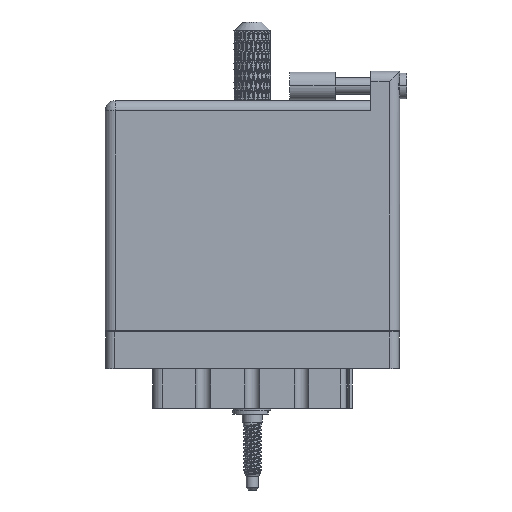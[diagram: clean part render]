
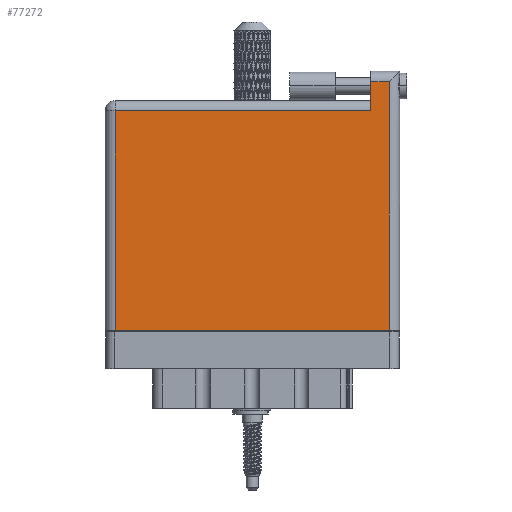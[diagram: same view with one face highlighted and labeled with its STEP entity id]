
A CAD part, front view. The second image highlights one B-rep face of the part: STEP entity #77272.
In plain terms, the highlighted face is planar.
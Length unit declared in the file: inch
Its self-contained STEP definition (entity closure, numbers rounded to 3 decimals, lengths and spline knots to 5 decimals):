
#939 = DIRECTION ( 'NONE',  ( 0., 0., -1. ) ) ;
#3342 = VECTOR ( 'NONE', #53919, 39.37008 ) ;
#4676 = VERTEX_POINT ( 'NONE', #93800 ) ;
#5300 = VERTEX_POINT ( 'NONE', #86890 ) ;
#16044 = ORIENTED_EDGE ( 'NONE', *, *, #45468, .T. ) ;
#17579 = EDGE_CURVE ( 'NONE', #5300, #91844, #90016, .T. ) ;
#21629 = VECTOR ( 'NONE', #67604, 39.37008 ) ;
#21723 = CARTESIAN_POINT ( 'NONE',  ( 1.811, 1.766, 0. ) ) ;
#23541 = VERTEX_POINT ( 'NONE', #57337 ) ;
#26443 = CARTESIAN_POINT ( 'NONE',  ( 0., 1.496, 0. ) ) ;
#26469 = VERTEX_POINT ( 'NONE', #27740 ) ;
#27039 = LINE ( 'NONE', #78316, #68382 ) ;
#27740 = CARTESIAN_POINT ( 'NONE',  ( 0.07, 0., 0. ) ) ;
#29326 = CARTESIAN_POINT ( 'NONE',  ( 0., 1.696, 0. ) ) ;
#29629 = FACE_OUTER_BOUND ( 'NONE', #103637, .T. ) ;
#32016 = ORIENTED_EDGE ( 'NONE', *, *, #65573, .T. ) ;
#35301 = LINE ( 'NONE', #66082, #44280 ) ;
#35376 = ORIENTED_EDGE ( 'NONE', *, *, #35683, .T. ) ;
#35683 = EDGE_CURVE ( 'NONE', #26469, #58102, #27039, .T. ) ;
#37629 = DIRECTION ( 'NONE',  ( -1., 0., 0. ) ) ;
#37657 = CARTESIAN_POINT ( 'NONE',  ( 1.938, 1.766, 0. ) ) ;
#44280 = VECTOR ( 'NONE', #48787, 39.37008 ) ;
#45468 = EDGE_CURVE ( 'NONE', #58102, #23541, #62739, .T. ) ;
#48787 = DIRECTION ( 'NONE',  ( 0., -1., 0. ) ) ;
#49992 = DIRECTION ( 'NONE',  ( -1., 0., 0. ) ) ;
#53919 = DIRECTION ( 'NONE',  ( 0., 1., 0. ) ) ;
#54588 = DIRECTION ( 'NONE',  ( 1., 0., 0. ) ) ;
#56483 = LINE ( 'NONE', #26443, #21629 ) ;
#57337 = CARTESIAN_POINT ( 'NONE',  ( 1.938, 1.696, 0. ) ) ;
#58102 = VERTEX_POINT ( 'NONE', #71157 ) ;
#62739 = LINE ( 'NONE', #37657, #3342 ) ;
#65550 = LINE ( 'NONE', #29326, #77062 ) ;
#65573 = EDGE_CURVE ( 'NONE', #4676, #26469, #35301, .T. ) ;
#66082 = CARTESIAN_POINT ( 'NONE',  ( 0.07, 0., 0. ) ) ;
#66584 = PLANE ( 'NONE',  #104550 ) ;
#67279 = CARTESIAN_POINT ( 'NONE',  ( 0., 1.566, 0. ) ) ;
#67604 = DIRECTION ( 'NONE',  ( -1., 0., 0. ) ) ;
#68084 = EDGE_CURVE ( 'NONE', #91844, #4676, #56483, .T. ) ;
#68382 = VECTOR ( 'NONE', #54588, 39.37008 ) ;
#71157 = CARTESIAN_POINT ( 'NONE',  ( 1.938, 0., 0. ) ) ;
#74999 = ORIENTED_EDGE ( 'NONE', *, *, #17579, .T. ) ;
#77062 = VECTOR ( 'NONE', #37629, 39.37008 ) ;
#77122 = VECTOR ( 'NONE', #104815, 39.37008 ) ;
#77272 = ADVANCED_FACE ( 'NONE', ( #29629 ), #66584, .F. ) ;
#78316 = CARTESIAN_POINT ( 'NONE',  ( 0., 0., 0. ) ) ;
#86890 = CARTESIAN_POINT ( 'NONE',  ( 1.811, 1.696, 0. ) ) ;
#90016 = LINE ( 'NONE', #21723, #77122 ) ;
#91844 = VERTEX_POINT ( 'NONE', #95416 ) ;
#93800 = CARTESIAN_POINT ( 'NONE',  ( 0.07, 1.496, 0. ) ) ;
#95416 = CARTESIAN_POINT ( 'NONE',  ( 1.811, 1.496, 0. ) ) ;
#101558 = ORIENTED_EDGE ( 'NONE', *, *, #68084, .T. ) ;
#102205 = ORIENTED_EDGE ( 'NONE', *, *, #104889, .T. ) ;
#103637 = EDGE_LOOP ( 'NONE', ( #35376, #16044, #102205, #74999, #101558, #32016 ) ) ;
#104550 = AXIS2_PLACEMENT_3D ( 'NONE', #67279, #939, #49992 ) ;
#104815 = DIRECTION ( 'NONE',  ( 0., -1., 0. ) ) ;
#104889 = EDGE_CURVE ( 'NONE', #23541, #5300, #65550, .T. ) ;
